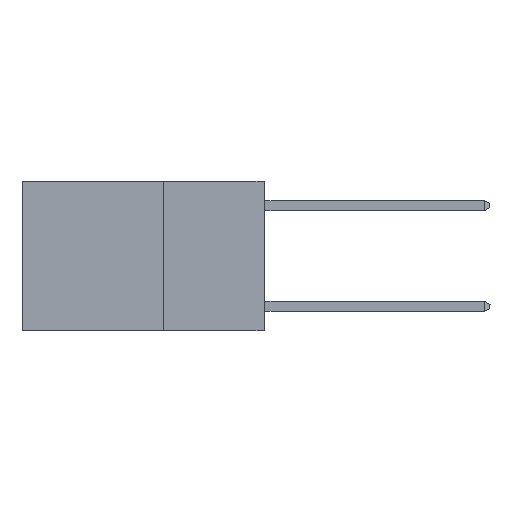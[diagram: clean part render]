
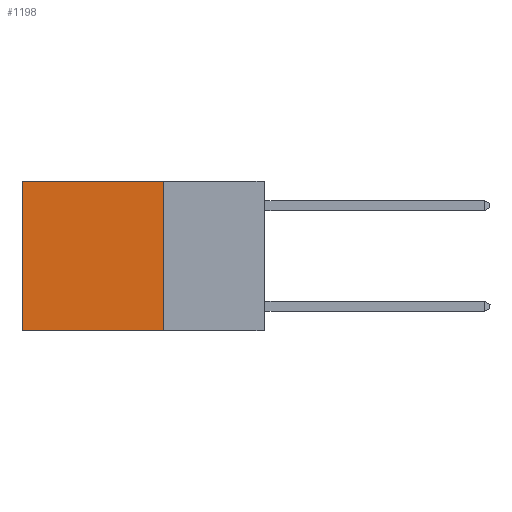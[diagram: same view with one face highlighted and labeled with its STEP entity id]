
A CAD part, left-side view. The second image highlights one B-rep face of the part: STEP entity #1198.
In plain terms, the highlighted planar face has unit normal (-1, 0, 0).
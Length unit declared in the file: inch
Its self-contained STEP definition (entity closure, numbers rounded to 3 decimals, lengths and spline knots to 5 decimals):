
#426 = LINE ( 'NONE', #11697, #7554 ) ;
#649 = EDGE_CURVE ( 'NONE', #5198, #8466, #8123, .T. ) ;
#872 = EDGE_CURVE ( 'NONE', #8997, #8466, #426, .T. ) ;
#1198 = ADVANCED_FACE ( 'NONE', ( #5723 ), #10727, .F. ) ;
#1288 = CARTESIAN_POINT ( 'NONE',  ( 0.2625, 0.6, -0.37 ) ) ;
#1674 = CARTESIAN_POINT ( 'NONE',  ( 0.2625, 0.6, 0. ) ) ;
#3421 = ORIENTED_EDGE ( 'NONE', *, *, #649, .T. ) ;
#3529 = VECTOR ( 'NONE', #9557, 39.37008 ) ;
#3584 = CARTESIAN_POINT ( 'NONE',  ( 0.2625, 0.25, 0. ) ) ;
#5198 = VERTEX_POINT ( 'NONE', #1674 ) ;
#5366 = EDGE_CURVE ( 'NONE', #8063, #8997, #10672, .T. ) ;
#5477 = CARTESIAN_POINT ( 'NONE',  ( 0.2625, 0.25, 0. ) ) ;
#5723 = FACE_OUTER_BOUND ( 'NONE', #7573, .T. ) ;
#5781 = ORIENTED_EDGE ( 'NONE', *, *, #872, .F. ) ;
#6121 = LINE ( 'NONE', #3584, #8388 ) ;
#6180 = DIRECTION ( 'NONE',  ( 0., 1., 0. ) ) ;
#6280 = EDGE_CURVE ( 'NONE', #8063, #5198, #6121, .T. ) ;
#6334 = DIRECTION ( 'NONE',  ( 0., 0., -1. ) ) ;
#6404 = CARTESIAN_POINT ( 'NONE',  ( 0.2625, 0.25, 0. ) ) ;
#6405 = DIRECTION ( 'NONE',  ( 0., 0., -1. ) ) ;
#6432 = CARTESIAN_POINT ( 'NONE',  ( 0.2625, 0.25, -0.37 ) ) ;
#7554 = VECTOR ( 'NONE', #9705, 39.37008 ) ;
#7573 = EDGE_LOOP ( 'NONE', ( #3421, #5781, #11012, #8016 ) ) ;
#7798 = AXIS2_PLACEMENT_3D ( 'NONE', #5477, #11590, #6334 ) ;
#7990 = VECTOR ( 'NONE', #6405, 39.37008 ) ;
#8016 = ORIENTED_EDGE ( 'NONE', *, *, #6280, .T. ) ;
#8063 = VERTEX_POINT ( 'NONE', #6404 ) ;
#8083 = CARTESIAN_POINT ( 'NONE',  ( 0.2625, 0.25, 0. ) ) ;
#8123 = LINE ( 'NONE', #9035, #3529 ) ;
#8388 = VECTOR ( 'NONE', #6180, 39.37008 ) ;
#8466 = VERTEX_POINT ( 'NONE', #1288 ) ;
#8997 = VERTEX_POINT ( 'NONE', #6432 ) ;
#9035 = CARTESIAN_POINT ( 'NONE',  ( 0.2625, 0.6, 0. ) ) ;
#9557 = DIRECTION ( 'NONE',  ( 0., 0., -1. ) ) ;
#9705 = DIRECTION ( 'NONE',  ( 0., 1., 0. ) ) ;
#10672 = LINE ( 'NONE', #8083, #7990 ) ;
#10727 = PLANE ( 'NONE',  #7798 ) ;
#11012 = ORIENTED_EDGE ( 'NONE', *, *, #5366, .F. ) ;
#11590 = DIRECTION ( 'NONE',  ( 1., 0., 0. ) ) ;
#11697 = CARTESIAN_POINT ( 'NONE',  ( 0.2625, 0.25, -0.37 ) ) ;
